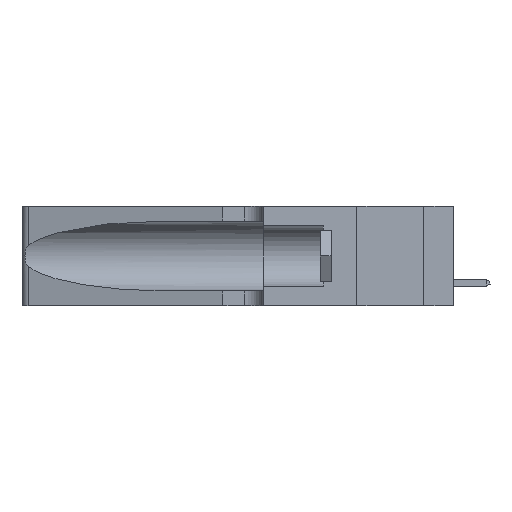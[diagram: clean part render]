
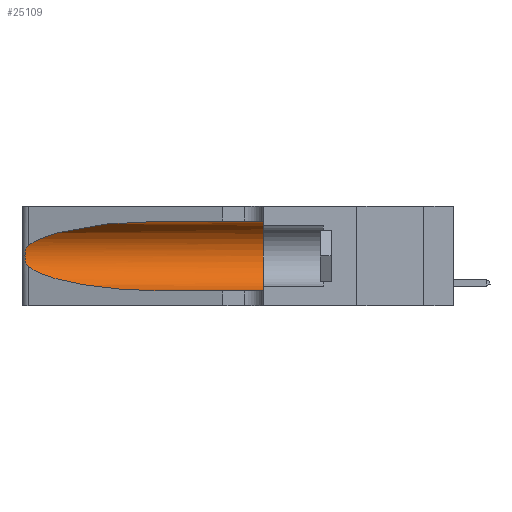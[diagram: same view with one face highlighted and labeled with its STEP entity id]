
A CAD part, left-side view. The second image highlights one B-rep face of the part: STEP entity #25109.
In plain terms, the highlighted cylindrical face has radius 3.308 mm (diameter 6.617 mm), a partial arc.
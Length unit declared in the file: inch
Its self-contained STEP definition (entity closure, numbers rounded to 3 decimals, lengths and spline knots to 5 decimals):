
#929 = CARTESIAN_POINT ( 'NONE',  ( 0.25789, 1.23486, 0.15765 ) ) ;
#1391 = EDGE_CURVE ( 'NONE', #25585, #5995, #21709, .T. ) ;
#1925 = CARTESIAN_POINT ( 'NONE',  ( 0.25487, 1.22718, 0.14631 ) ) ;
#1987 = LINE ( 'NONE', #32625, #47317 ) ;
#2495 = ORIENTED_EDGE ( 'NONE', *, *, #21673, .T. ) ;
#3381 = CIRCLE ( 'NONE', #37047, 0.13025 ) ;
#3428 = CARTESIAN_POINT ( 'NONE',  ( 0.1305, 0.35, 0.31525 ) ) ;
#4008 = CARTESIAN_POINT ( 'NONE',  ( 0.25854, 1.2359, 0.20912 ) ) ;
#4209 = ORIENTED_EDGE ( 'NONE', *, *, #1391, .F. ) ;
#5054 = CARTESIAN_POINT ( 'NONE',  ( 0.1305, 0.72297, 0.05475 ) ) ;
#5591 = CARTESIAN_POINT ( 'NONE',  ( 0.25487, 1.22718, 0.14631 ) ) ;
#5778 = EDGE_CURVE ( 'NONE', #25585, #28652, #38063, .T. ) ;
#5995 = VERTEX_POINT ( 'NONE', #3428 ) ;
#6291 = CARTESIAN_POINT ( 'NONE',  ( 0.2373, 1.15595, 0.08982 ) ) ;
#6520 = DIRECTION ( 'NONE',  ( 0., 0., 1. ) ) ;
#7670 = CARTESIAN_POINT ( 'NONE',  ( 0.25787, 1.23484, 0.2124 ) ) ;
#9599 = CARTESIAN_POINT ( 'NONE',  ( 0.1305, 0.72297, 0.05475 ) ) ;
#9610 =( BOUNDED_CURVE ( )  B_SPLINE_CURVE ( 3, ( #1925, #6291, #44483, #9599 ),
 .UNSPECIFIED., .F., .F. ) 
 B_SPLINE_CURVE_WITH_KNOTS ( ( 4, 4 ),
 ( 3.44316, 4.71239 ),
 .UNSPECIFIED. ) 
 CURVE ( )  GEOMETRIC_REPRESENTATION_ITEM ( )  RATIONAL_B_SPLINE_CURVE ( ( 1., 0.87, 0.87, 1. ) ) 
 REPRESENTATION_ITEM ( '' )  );
#13837 = EDGE_CURVE ( 'NONE', #5995, #18440, #3381, .T. ) ;
#14049 = CARTESIAN_POINT ( 'NONE',  ( 0.25487, 1.22718, 0.22369 ) ) ;
#14686 = FACE_OUTER_BOUND ( 'NONE', #38588, .T. ) ;
#15095 = CARTESIAN_POINT ( 'NONE',  ( 0.25555, 1.22994, 0.2215 ) ) ;
#15259 = CARTESIAN_POINT ( 'NONE',  ( 0.25639, 1.23184, 0.21858 ) ) ;
#15593 = EDGE_CURVE ( 'NONE', #21471, #20484, #9610, .T. ) ;
#16555 = ORIENTED_EDGE ( 'NONE', *, *, #15593, .T. ) ;
#16895 = B_SPLINE_CURVE_WITH_KNOTS ( 'NONE', 3,
 ( #44883, #15095, #15259, #7670, #4008, #46002, #42623, #23704, #19734, #27395, #929, #35231, #39748, #5591 ),
 .UNSPECIFIED., .F., .F.,
 ( 4, 2, 2, 2, 2, 2, 4 ),
 ( 0., 0.00027, 0.00053, 0.00107, 0.0016, 0.00187, 0.00214 ),
 .UNSPECIFIED. ) ;
#17009 = DIRECTION ( 'NONE',  ( 0., -1., 0. ) ) ;
#17181 = AXIS2_PLACEMENT_3D ( 'NONE', #36004, #17009, #44432 ) ;
#18288 = ORIENTED_EDGE ( 'NONE', *, *, #13837, .F. ) ;
#18440 = VERTEX_POINT ( 'NONE', #31706 ) ;
#19734 = CARTESIAN_POINT ( 'NONE',  ( 0.26017, 1.23833, 0.17102 ) ) ;
#20484 = VERTEX_POINT ( 'NONE', #5054 ) ;
#21471 = VERTEX_POINT ( 'NONE', #28345 ) ;
#21673 = EDGE_CURVE ( 'NONE', #28652, #21471, #16895, .T. ) ;
#21709 = LINE ( 'NONE', #28886, #27041 ) ;
#22712 = CARTESIAN_POINT ( 'NONE',  ( 0.1305, 0.72297, 0.31525 ) ) ;
#23389 = ORIENTED_EDGE ( 'NONE', *, *, #5778, .T. ) ;
#23704 = CARTESIAN_POINT ( 'NONE',  ( 0.26075, 1.23896, 0.178 ) ) ;
#25109 = ADVANCED_FACE ( 'NONE', ( #14686 ), #32575, .F. ) ;
#25445 = DIRECTION ( 'NONE',  ( 0., 1., 0. ) ) ;
#25585 = VERTEX_POINT ( 'NONE', #35820 ) ;
#26867 = EDGE_CURVE ( 'NONE', #20484, #18440, #1987, .T. ) ;
#27041 = VECTOR ( 'NONE', #47398, 39.37008 ) ;
#27395 = CARTESIAN_POINT ( 'NONE',  ( 0.25856, 1.23593, 0.16098 ) ) ;
#28345 = CARTESIAN_POINT ( 'NONE',  ( 0.25487, 1.22718, 0.14631 ) ) ;
#28652 = VERTEX_POINT ( 'NONE', #14049 ) ;
#28886 = CARTESIAN_POINT ( 'NONE',  ( 0.1305, 1.61858, 0.31525 ) ) ;
#28970 = DIRECTION ( 'NONE',  ( 0., -1., 0. ) ) ;
#31706 = CARTESIAN_POINT ( 'NONE',  ( 0.1305, 0.35, 0.05475 ) ) ;
#32575 = CYLINDRICAL_SURFACE ( 'NONE', #17181, 0.13025 ) ;
#32625 = CARTESIAN_POINT ( 'NONE',  ( 0.1305, 1.61858, 0.05475 ) ) ;
#33477 = CARTESIAN_POINT ( 'NONE',  ( 0.1305, 0.35, 0.185 ) ) ;
#35231 = CARTESIAN_POINT ( 'NONE',  ( 0.25639, 1.23186, 0.15144 ) ) ;
#35820 = CARTESIAN_POINT ( 'NONE',  ( 0.1305, 0.72297, 0.31525 ) ) ;
#36004 = CARTESIAN_POINT ( 'NONE',  ( 0.1305, 1.61858, 0.185 ) ) ;
#37047 = AXIS2_PLACEMENT_3D ( 'NONE', #33477, #25445, #6520 ) ;
#38050 = CARTESIAN_POINT ( 'NONE',  ( 0.18966, 0.96281, 0.31525 ) ) ;
#38063 =( BOUNDED_CURVE ( )  B_SPLINE_CURVE ( 3, ( #22712, #38050, #41429, #49101 ),
 .UNSPECIFIED., .F., .T. ) 
 B_SPLINE_CURVE_WITH_KNOTS ( ( 4, 4 ),
 ( 1.5708, 2.84003 ),
 .UNSPECIFIED. ) 
 CURVE ( )  GEOMETRIC_REPRESENTATION_ITEM ( )  RATIONAL_B_SPLINE_CURVE ( ( 1., 0.87, 0.87, 1. ) ) 
 REPRESENTATION_ITEM ( '' )  );
#38588 = EDGE_LOOP ( 'NONE', ( #23389, #2495, #16555, #48642, #18288, #4209 ) ) ;
#39748 = CARTESIAN_POINT ( 'NONE',  ( 0.25555, 1.22993, 0.14849 ) ) ;
#41429 = CARTESIAN_POINT ( 'NONE',  ( 0.2373, 1.15595, 0.28018 ) ) ;
#42623 = CARTESIAN_POINT ( 'NONE',  ( 0.26075, 1.23896, 0.19203 ) ) ;
#44432 = DIRECTION ( 'NONE',  ( 0., 0., -1. ) ) ;
#44483 = CARTESIAN_POINT ( 'NONE',  ( 0.18966, 0.96281, 0.05475 ) ) ;
#44883 = CARTESIAN_POINT ( 'NONE',  ( 0.25487, 1.22718, 0.22369 ) ) ;
#46002 = CARTESIAN_POINT ( 'NONE',  ( 0.26018, 1.23835, 0.19895 ) ) ;
#47317 = VECTOR ( 'NONE', #28970, 39.37008 ) ;
#47398 = DIRECTION ( 'NONE',  ( 0., -1., 0. ) ) ;
#48642 = ORIENTED_EDGE ( 'NONE', *, *, #26867, .T. ) ;
#49101 = CARTESIAN_POINT ( 'NONE',  ( 0.25487, 1.22718, 0.22369 ) ) ;
